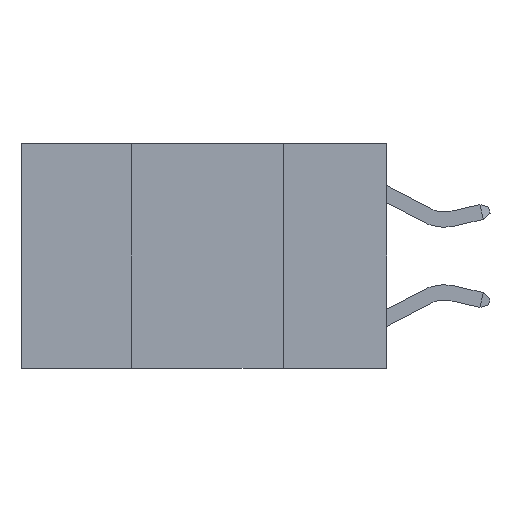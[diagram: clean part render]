
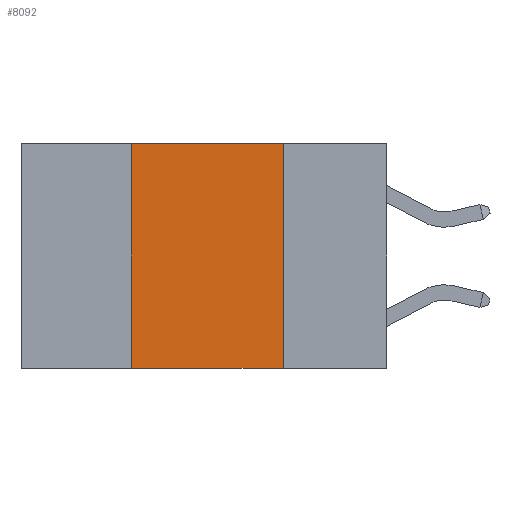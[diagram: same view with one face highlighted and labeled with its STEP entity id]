
A CAD part, left-side view. The second image highlights one B-rep face of the part: STEP entity #8092.
In plain terms, the highlighted planar face has unit normal (-1, 0, 0).
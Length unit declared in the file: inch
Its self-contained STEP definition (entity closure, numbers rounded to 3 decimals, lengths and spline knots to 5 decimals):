
#1198 = DIRECTION ( 'NONE',  ( 0., -1., 0. ) ) ;
#1597 = CARTESIAN_POINT ( 'NONE',  ( 0., 0.42, 0. ) ) ;
#1740 = ORIENTED_EDGE ( 'NONE', *, *, #9369, .T. ) ;
#2221 = VECTOR ( 'NONE', #1198, 39.37008 ) ;
#2507 = VERTEX_POINT ( 'NONE', #1597 ) ;
#2894 = CARTESIAN_POINT ( 'NONE',  ( 0., 0.17, 0. ) ) ;
#3060 = EDGE_CURVE ( 'NONE', #11974, #3684, #10630, .T. ) ;
#3099 = VECTOR ( 'NONE', #10589, 39.37008 ) ;
#3684 = VERTEX_POINT ( 'NONE', #17382 ) ;
#4721 = CARTESIAN_POINT ( 'NONE',  ( 0., 0.42, -0.37 ) ) ;
#4869 = EDGE_CURVE ( 'NONE', #10463, #2507, #15363, .T. ) ;
#4887 = ORIENTED_EDGE ( 'NONE', *, *, #11028, .F. ) ;
#5436 = PLANE ( 'NONE',  #13783 ) ;
#5711 = ORIENTED_EDGE ( 'NONE', *, *, #4869, .F. ) ;
#6794 = DIRECTION ( 'NONE',  ( 0., 0., -1. ) ) ;
#6965 = EDGE_LOOP ( 'NONE', ( #7606, #4887, #5711, #1740 ) ) ;
#7606 = ORIENTED_EDGE ( 'NONE', *, *, #3060, .F. ) ;
#8092 = ADVANCED_FACE ( 'NONE', ( #12743 ), #5436, .F. ) ;
#9094 = CARTESIAN_POINT ( 'NONE',  ( 0., 0.6, -0.37 ) ) ;
#9154 = DIRECTION ( 'NONE',  ( 0., -1., 0. ) ) ;
#9265 = CARTESIAN_POINT ( 'NONE',  ( 0., 0.6, 0. ) ) ;
#9369 = EDGE_CURVE ( 'NONE', #10463, #3684, #17306, .T. ) ;
#9492 = CARTESIAN_POINT ( 'NONE',  ( 0., 0.42, 0. ) ) ;
#10463 = VERTEX_POINT ( 'NONE', #4721 ) ;
#10589 = DIRECTION ( 'NONE',  ( 0., 0., -1. ) ) ;
#10630 = LINE ( 'NONE', #13269, #3099 ) ;
#10742 = CARTESIAN_POINT ( 'NONE',  ( 0., 0.6, 0. ) ) ;
#10819 = DIRECTION ( 'NONE',  ( 0., 0., 1. ) ) ;
#11028 = EDGE_CURVE ( 'NONE', #2507, #11974, #16021, .T. ) ;
#11974 = VERTEX_POINT ( 'NONE', #2894 ) ;
#12250 = VECTOR ( 'NONE', #10819, 39.37008 ) ;
#12743 = FACE_OUTER_BOUND ( 'NONE', #6965, .T. ) ;
#13269 = CARTESIAN_POINT ( 'NONE',  ( 0., 0.17, 0. ) ) ;
#13774 = VECTOR ( 'NONE', #9154, 39.37008 ) ;
#13783 = AXIS2_PLACEMENT_3D ( 'NONE', #10742, #14755, #6794 ) ;
#14755 = DIRECTION ( 'NONE',  ( 1., 0., 0. ) ) ;
#15363 = LINE ( 'NONE', #9492, #12250 ) ;
#16021 = LINE ( 'NONE', #9265, #2221 ) ;
#17306 = LINE ( 'NONE', #9094, #13774 ) ;
#17382 = CARTESIAN_POINT ( 'NONE',  ( 0., 0.17, -0.37 ) ) ;
